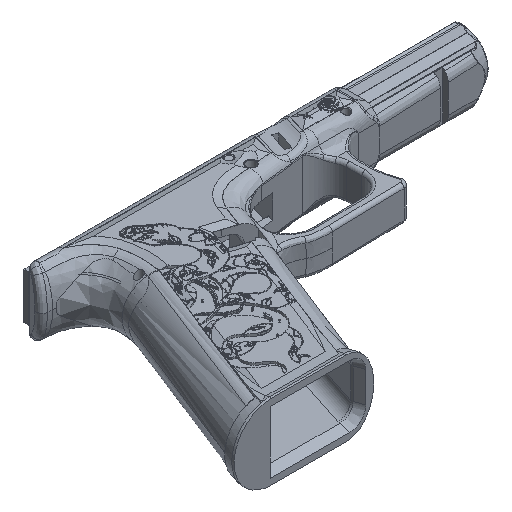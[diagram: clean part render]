
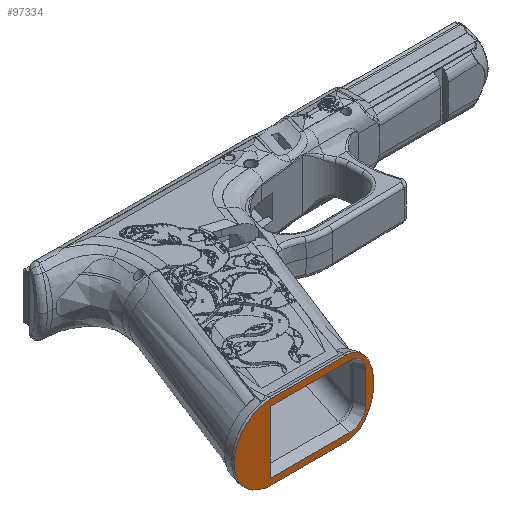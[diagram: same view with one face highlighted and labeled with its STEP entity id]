
A CAD part, isometric view. The second image highlights one B-rep face of the part: STEP entity #97334.
In plain terms, the highlighted planar face has unit normal (0, -1, 0).
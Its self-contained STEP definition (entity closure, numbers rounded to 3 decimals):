
#265=ELLIPSE('',#98559,16.,11.5);
#580=FACE_BOUND('',#12181,.T.);
#959=CIRCLE('',#98556,16.);
#1503=PLANE('',#98558);
#6725=FACE_OUTER_BOUND('',#12180,.T.);
#12180=EDGE_LOOP('',(#87226,#87227,#87228,#87229));
#12181=EDGE_LOOP('',(#87230,#87231,#87232,#87233,#87234,#87235));
#21761=LINE('',#223763,#27029);
#21763=LINE('',#223767,#27031);
#21766=LINE('',#223803,#27034);
#21770=LINE('',#223839,#27038);
#21829=LINE('',#230455,#27097);
#21830=LINE('',#230457,#27098);
#27029=VECTOR('',#105881,10.);
#27031=VECTOR('',#105885,10.);
#27034=VECTOR('',#105890,10.);
#27038=VECTOR('',#105896,10.);
#27097=VECTOR('',#106121,10.);
#27098=VECTOR('',#106122,10.);
#32037=B_SPLINE_CURVE_WITH_KNOTS('',3,(#223794,#223795,#223796,#223797,
#223798,#223799),.UNSPECIFIED.,.F.,.F.,(4,1,1,4),(-1.571,-1.122,
-0.673,0.),.UNSPECIFIED.);
#32038=B_SPLINE_CURVE_WITH_KNOTS('',3,(#223830,#223831,#223832,#223833,
#223834,#223835),.UNSPECIFIED.,.F.,.F.,(4,1,1,4),(0.,
0.673,1.122,1.571),.UNSPECIFIED.);
#42028=VERTEX_POINT('',#223760);
#42029=VERTEX_POINT('',#223762);
#42030=VERTEX_POINT('',#223766);
#42031=VERTEX_POINT('',#223793);
#42032=VERTEX_POINT('',#223802);
#42033=VERTEX_POINT('',#223829);
#42163=VERTEX_POINT('',#230447);
#42164=VERTEX_POINT('',#230449);
#42165=VERTEX_POINT('',#230454);
#42166=VERTEX_POINT('',#230456);
#57019=EDGE_CURVE('',#42028,#42029,#21761,.T.);
#57021=EDGE_CURVE('',#42029,#42030,#21763,.T.);
#57023=EDGE_CURVE('',#42030,#42031,#32037,.T.);
#57025=EDGE_CURVE('',#42031,#42032,#21766,.T.);
#57027=EDGE_CURVE('',#42032,#42033,#32038,.T.);
#57030=EDGE_CURVE('',#42033,#42028,#21770,.T.);
#57247=EDGE_CURVE('',#42164,#42163,#959,.T.);
#57250=EDGE_CURVE('',#42165,#42164,#21829,.T.);
#57251=EDGE_CURVE('',#42163,#42166,#21830,.T.);
#57252=EDGE_CURVE('',#42166,#42165,#265,.T.);
#87226=ORIENTED_EDGE('',*,*,#57250,.T.);
#87227=ORIENTED_EDGE('',*,*,#57247,.T.);
#87228=ORIENTED_EDGE('',*,*,#57251,.T.);
#87229=ORIENTED_EDGE('',*,*,#57252,.T.);
#87230=ORIENTED_EDGE('',*,*,#57030,.F.);
#87231=ORIENTED_EDGE('',*,*,#57027,.F.);
#87232=ORIENTED_EDGE('',*,*,#57025,.F.);
#87233=ORIENTED_EDGE('',*,*,#57023,.F.);
#87234=ORIENTED_EDGE('',*,*,#57021,.F.);
#87235=ORIENTED_EDGE('',*,*,#57019,.F.);
#97334=ADVANCED_FACE('',(#6725,#580),#1503,.T.);
#98556=AXIS2_PLACEMENT_3D('',#230450,#106114,#106115);
#98558=AXIS2_PLACEMENT_3D('',#230453,#106119,#106120);
#98559=AXIS2_PLACEMENT_3D('',#230458,#106123,#106124);
#105881=DIRECTION('',(0.,0.,-1.));
#105885=DIRECTION('',(1.,0.,0.));
#105890=DIRECTION('',(0.,0.,1.));
#105896=DIRECTION('',(-1.,0.,0.));
#106114=DIRECTION('center_axis',(0.,-1.,0.));
#106115=DIRECTION('ref_axis',(1.,0.,0.));
#106119=DIRECTION('center_axis',(0.,-1.,0.));
#106120=DIRECTION('ref_axis',(1.,0.,0.));
#106121=DIRECTION('',(-1.,0.,0.));
#106122=DIRECTION('',(1.,0.,0.));
#106123=DIRECTION('center_axis',(0.,-1.,0.));
#106124=DIRECTION('ref_axis',(0.,0.,-1.));
#223760=CARTESIAN_POINT('',(-1.539,-105.,13.25));
#223762=CARTESIAN_POINT('',(-1.539,-105.,-13.25));
#223763=CARTESIAN_POINT('',(-1.539,-105.,-5.875));
#223766=CARTESIAN_POINT('',(32.201,-105.,-13.25));
#223767=CARTESIAN_POINT('',(5.275,-105.,-13.25));
#223793=CARTESIAN_POINT('',(39.169,-105.,-6.55));
#223794=CARTESIAN_POINT('Ctrl Pts',(32.201,-105.,-13.25));
#223795=CARTESIAN_POINT('Ctrl Pts',(33.232,-105.,-13.25));
#223796=CARTESIAN_POINT('Ctrl Pts',(35.291,-105.,-12.802));
#223797=CARTESIAN_POINT('Ctrl Pts',(38.229,-105.,-10.589));
#223798=CARTESIAN_POINT('Ctrl Pts',(39.169,-105.,-8.071));
#223799=CARTESIAN_POINT('Ctrl Pts',(39.169,-105.,-6.55));
#223802=CARTESIAN_POINT('',(39.169,-105.,6.55));
#223803=CARTESIAN_POINT('',(39.169,-105.,3.275));
#223829=CARTESIAN_POINT('',(32.201,-105.,13.25));
#223830=CARTESIAN_POINT('Ctrl Pts',(39.169,-105.,6.55));
#223831=CARTESIAN_POINT('Ctrl Pts',(39.169,-105.,8.071));
#223832=CARTESIAN_POINT('Ctrl Pts',(38.229,-105.,10.589));
#223833=CARTESIAN_POINT('Ctrl Pts',(35.291,-105.,12.802));
#223834=CARTESIAN_POINT('Ctrl Pts',(33.232,-105.,13.25));
#223835=CARTESIAN_POINT('Ctrl Pts',(32.201,-105.,13.25));
#223839=CARTESIAN_POINT('',(5.275,-105.,13.25));
#230447=CARTESIAN_POINT('',(-1.,-105.,-16.));
#230449=CARTESIAN_POINT('',(-1.,-105.,16.));
#230450=CARTESIAN_POINT('Origin',(-1.,-105.,0.));
#230453=CARTESIAN_POINT('Origin',(12.75,-105.,0.));
#230454=CARTESIAN_POINT('',(31.,-105.,16.));
#230455=CARTESIAN_POINT('',(32.,-105.,16.));
#230456=CARTESIAN_POINT('',(31.,-105.,-16.));
#230457=CARTESIAN_POINT('',(-1.,-105.,-16.));
#230458=CARTESIAN_POINT('Origin',(31.,-105.,0.));
